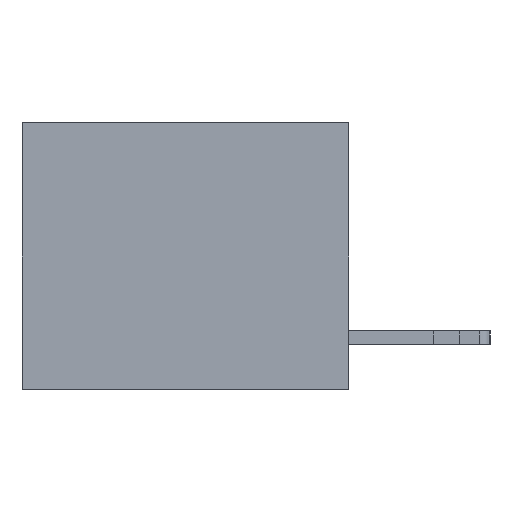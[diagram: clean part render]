
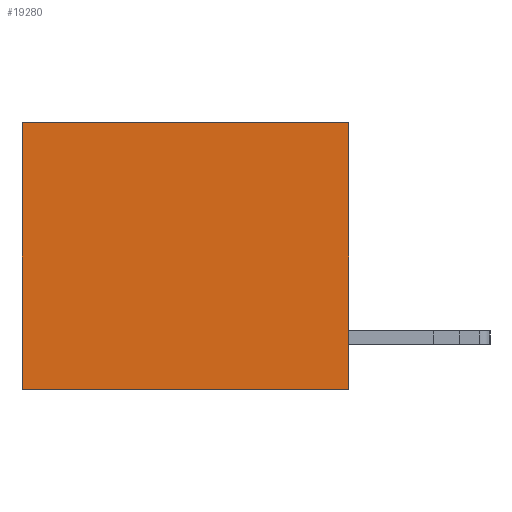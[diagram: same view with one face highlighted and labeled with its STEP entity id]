
A CAD part, left-side view. The second image highlights one B-rep face of the part: STEP entity #19280.
In plain terms, the highlighted planar face has unit normal (-1, 0, 0).
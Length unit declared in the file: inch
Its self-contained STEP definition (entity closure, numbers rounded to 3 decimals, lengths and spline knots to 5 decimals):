
#758 = EDGE_CURVE ( 'NONE', #1484, #8019, #4478, .T. ) ;
#1484 = VERTEX_POINT ( 'NONE', #12901 ) ;
#1502 = DIRECTION ( 'NONE',  ( 0., 0., -1. ) ) ;
#3665 = CARTESIAN_POINT ( 'NONE',  ( 0.3165, 0.6, -0.49 ) ) ;
#3735 = DIRECTION ( 'NONE',  ( 0., 0., -1. ) ) ;
#4437 = LINE ( 'NONE', #3665, #18625 ) ;
#4478 = LINE ( 'NONE', #8014, #9028 ) ;
#5369 = DIRECTION ( 'NONE',  ( 0., 0., -1. ) ) ;
#5435 = VECTOR ( 'NONE', #18584, 39.37008 ) ;
#6245 = FACE_OUTER_BOUND ( 'NONE', #8367, .T. ) ;
#6485 = CARTESIAN_POINT ( 'NONE',  ( 0.3165, 0.6, -0.49 ) ) ;
#8014 = CARTESIAN_POINT ( 'NONE',  ( 0.3165, 0., -0.49 ) ) ;
#8019 = VERTEX_POINT ( 'NONE', #6485 ) ;
#8073 = CARTESIAN_POINT ( 'NONE',  ( 0.3165, 0., -0.49 ) ) ;
#8284 = ORIENTED_EDGE ( 'NONE', *, *, #758, .F. ) ;
#8367 = EDGE_LOOP ( 'NONE', ( #12730, #8284, #20734, #10144 ) ) ;
#8934 = CARTESIAN_POINT ( 'NONE',  ( 0.3165, 0.6, 0. ) ) ;
#8951 = EDGE_CURVE ( 'NONE', #9821, #15178, #17568, .T. ) ;
#9028 = VECTOR ( 'NONE', #20751, 39.37008 ) ;
#9292 = CARTESIAN_POINT ( 'NONE',  ( 0.3165, 0., 0. ) ) ;
#9821 = VERTEX_POINT ( 'NONE', #9292 ) ;
#10144 = ORIENTED_EDGE ( 'NONE', *, *, #8951, .T. ) ;
#10745 = EDGE_CURVE ( 'NONE', #9821, #1484, #13973, .T. ) ;
#12252 = CARTESIAN_POINT ( 'NONE',  ( 0.3165, 0., 0. ) ) ;
#12730 = ORIENTED_EDGE ( 'NONE', *, *, #14273, .T. ) ;
#12901 = CARTESIAN_POINT ( 'NONE',  ( 0.3165, 0., -0.49 ) ) ;
#13337 = CARTESIAN_POINT ( 'NONE',  ( 0.3165, 0., -0.49 ) ) ;
#13973 = LINE ( 'NONE', #8073, #20584 ) ;
#14273 = EDGE_CURVE ( 'NONE', #15178, #8019, #4437, .T. ) ;
#15042 = PLANE ( 'NONE',  #15644 ) ;
#15178 = VERTEX_POINT ( 'NONE', #8934 ) ;
#15644 = AXIS2_PLACEMENT_3D ( 'NONE', #13337, #16679, #5369 ) ;
#16679 = DIRECTION ( 'NONE',  ( 1., 0., 0. ) ) ;
#17568 = LINE ( 'NONE', #12252, #5435 ) ;
#18584 = DIRECTION ( 'NONE',  ( 0., 1., 0. ) ) ;
#18625 = VECTOR ( 'NONE', #3735, 39.37008 ) ;
#19280 = ADVANCED_FACE ( 'NONE', ( #6245 ), #15042, .F. ) ;
#20584 = VECTOR ( 'NONE', #1502, 39.37008 ) ;
#20734 = ORIENTED_EDGE ( 'NONE', *, *, #10745, .F. ) ;
#20751 = DIRECTION ( 'NONE',  ( 0., 1., 0. ) ) ;
